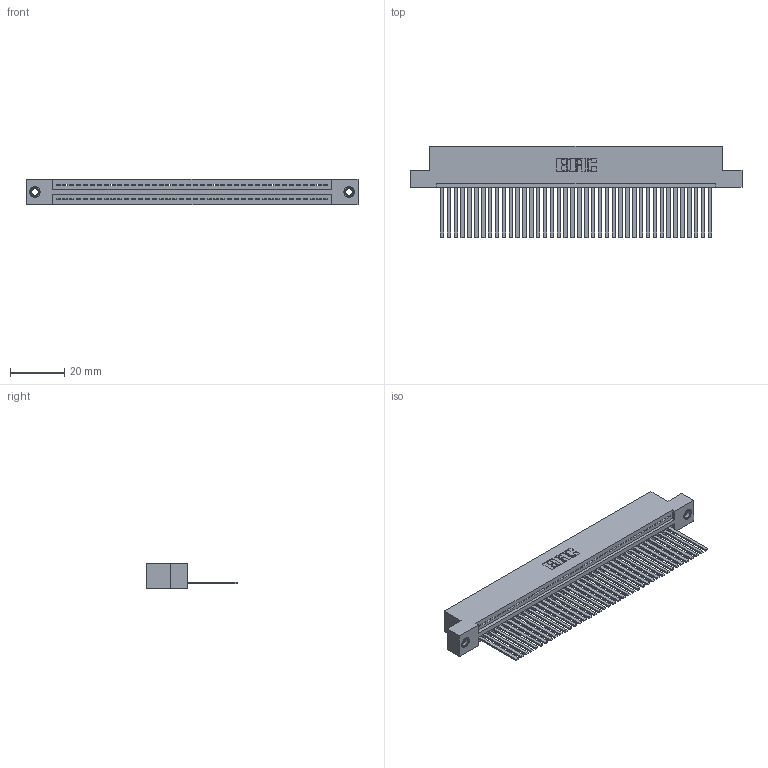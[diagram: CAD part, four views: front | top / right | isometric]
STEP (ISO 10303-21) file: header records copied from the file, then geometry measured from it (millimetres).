
FILE_DESCRIPTION (( 'STEP AP203' ), '1' );
FILE_NAME ('395-040-544-107.STEP', '2019-10-22T05:51:32', ( '' ), ( '' ), 'SwSTEP 2.0', 'SolidWorks 2016', '' );
FILE_SCHEMA (( 'CONFIG_CONTROL_DESIGN' ));
Length unit declared in the file: inch
Products named in the file (4): 345-250-001_345-250-005-103; 395-040-544-107; 345-292-001_345-293-144; 345 Part_Flush Mounting Lugs - 0.156 Dia-TI
Assembly tree (43 placements, depth 2):
  395-040-544-107
    345 Part_Flush Mounting Lugs - 0.156 Dia-TI
    345-292-001_345-293-144  x40
    345-250-001_345-250-005-103  x2
Bounding box: 122.81 x 33.96 x 9.4 mm (x, y, z)
Volume: 12097.9 mm3; surface area: 17473.1 mm2
Topology: 43 solids, 43 shells, 2266 faces, 6797 edges, 4470 vertices
Faces by surface type: plane 1552, cylinder 698, cone 12, torus 4
Entity records: 31376 total; most frequent: CARTESIAN_POINT 5415, ORIENTED_EDGE 5382, DIRECTION 4757, EDGE_CURVE 2691, VECTOR 2383, LINE 2383, VERTEX_POINT 1788, AXIS2_PLACEMENT_3D 1187
